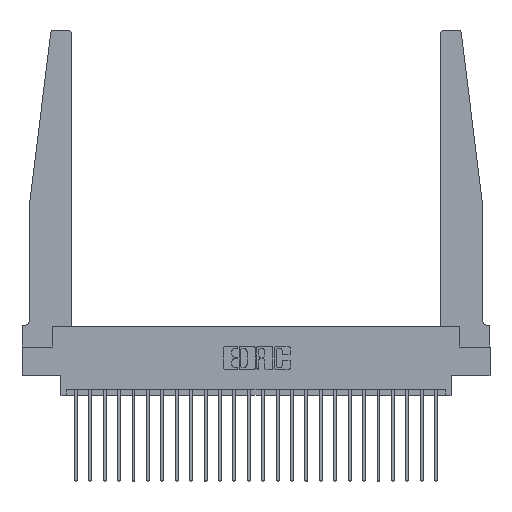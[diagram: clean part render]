
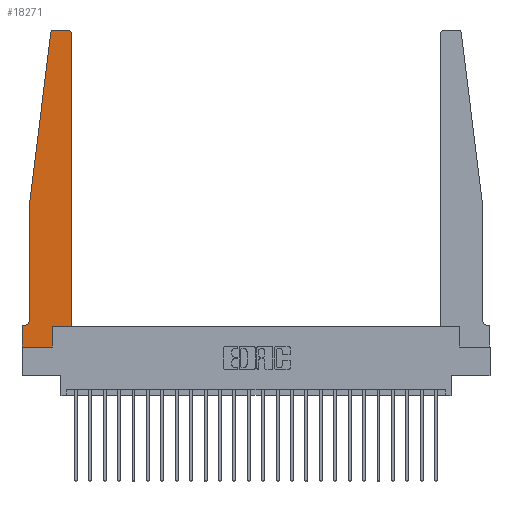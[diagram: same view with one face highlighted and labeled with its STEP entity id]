
A CAD part, top view. The second image highlights one B-rep face of the part: STEP entity #18271.
In plain terms, the highlighted planar face has unit normal (0, 0, 1).
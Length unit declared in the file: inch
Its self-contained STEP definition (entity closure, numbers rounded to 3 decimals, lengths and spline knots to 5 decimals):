
#28 = VECTOR ( 'NONE', #13518, 39.37008 ) ;
#269 = CARTESIAN_POINT ( 'NONE',  ( 0.24675, 2.72367, 0.37 ) ) ;
#648 = ORIENTED_EDGE ( 'NONE', *, *, #5859, .T. ) ;
#719 = CARTESIAN_POINT ( 'NONE',  ( 0., 0., 0.37 ) ) ;
#988 = DIRECTION ( 'NONE',  ( -1., 0., 0. ) ) ;
#1065 = EDGE_CURVE ( 'NONE', #1542, #18862, #12877, .T. ) ;
#1281 = CARTESIAN_POINT ( 'NONE',  ( 0.065, 1.25, 0.37 ) ) ;
#1542 = VERTEX_POINT ( 'NONE', #18149 ) ;
#1634 = CARTESIAN_POINT ( 'NONE',  ( 0.065, 0.1875, 0.37 ) ) ;
#1812 = ORIENTED_EDGE ( 'NONE', *, *, #22918, .T. ) ;
#2038 = EDGE_CURVE ( 'NONE', #8043, #19866, #11413, .T. ) ;
#2056 = EDGE_CURVE ( 'NONE', #17575, #8043, #7572, .T. ) ;
#2084 = ORIENTED_EDGE ( 'NONE', *, *, #17867, .T. ) ;
#2515 = DIRECTION ( 'NONE',  ( 0., 0., 1. ) ) ;
#3106 = VERTEX_POINT ( 'NONE', #269 ) ;
#3423 = DIRECTION ( 'NONE',  ( 0., -1., 0. ) ) ;
#3933 = CARTESIAN_POINT ( 'NONE',  ( 0., 0., 0.37 ) ) ;
#4007 = VECTOR ( 'NONE', #5927, 39.37008 ) ;
#4146 = VECTOR ( 'NONE', #988, 39.37008 ) ;
#4293 = CARTESIAN_POINT ( 'NONE',  ( 0.015, 0.2375, 0.37 ) ) ;
#4571 = ORIENTED_EDGE ( 'NONE', *, *, #20553, .T. ) ;
#5697 = FACE_OUTER_BOUND ( 'NONE', #13056, .T. ) ;
#5859 = EDGE_CURVE ( 'NONE', #18862, #10636, #10485, .T. ) ;
#5927 = DIRECTION ( 'NONE',  ( 1., 0., 0. ) ) ;
#6132 = ORIENTED_EDGE ( 'NONE', *, *, #16201, .T. ) ;
#6278 = DIRECTION ( 'NONE',  ( 1., 0., 0. ) ) ;
#6627 = DIRECTION ( 'NONE',  ( 0., 1., 0. ) ) ;
#6885 = CARTESIAN_POINT ( 'NONE',  ( 0.27653, 2.75, 0.37 ) ) ;
#7199 = ORIENTED_EDGE ( 'NONE', *, *, #8914, .T. ) ;
#7244 = ORIENTED_EDGE ( 'NONE', *, *, #2038, .T. ) ;
#7515 = LINE ( 'NONE', #18513, #19629 ) ;
#7572 = LINE ( 'NONE', #3933, #28 ) ;
#7849 = ORIENTED_EDGE ( 'NONE', *, *, #2056, .T. ) ;
#8014 = CARTESIAN_POINT ( 'NONE',  ( 0.425, 2.72, 0.37 ) ) ;
#8043 = VERTEX_POINT ( 'NONE', #719 ) ;
#8111 = AXIS2_PLACEMENT_3D ( 'NONE', #4293, #11889, #19625 ) ;
#8157 = CARTESIAN_POINT ( 'NONE',  ( 0.395, 2.72, 0.37 ) ) ;
#8914 = EDGE_CURVE ( 'NONE', #11824, #17312, #10185, .T. ) ;
#10185 = CIRCLE ( 'NONE', #19604, 0.03 ) ;
#10283 = VECTOR ( 'NONE', #17275, 39.37008 ) ;
#10485 = CIRCLE ( 'NONE', #8111, 0.05 ) ;
#10636 = VERTEX_POINT ( 'NONE', #20824 ) ;
#11190 = DIRECTION ( 'NONE',  ( 0., 0., 1. ) ) ;
#11413 = LINE ( 'NONE', #20982, #4007 ) ;
#11824 = VERTEX_POINT ( 'NONE', #8014 ) ;
#11889 = DIRECTION ( 'NONE',  ( 0., 0., -1. ) ) ;
#11905 = AXIS2_PLACEMENT_3D ( 'NONE', #17106, #11190, #18698 ) ;
#12877 = LINE ( 'NONE', #1281, #14696 ) ;
#12931 = VECTOR ( 'NONE', #15034, 39.37008 ) ;
#12952 = CARTESIAN_POINT ( 'NONE',  ( 0.425, 0.18, 0.37 ) ) ;
#13056 = EDGE_LOOP ( 'NONE', ( #13083, #1812, #18949, #24376, #648, #6132, #7849, #7244, #15143, #4571, #2084, #7199 ) ) ;
#13083 = ORIENTED_EDGE ( 'NONE', *, *, #21608, .T. ) ;
#13289 = PLANE ( 'NONE',  #11905 ) ;
#13518 = DIRECTION ( 'NONE',  ( 0., -1., 0. ) ) ;
#13530 = EDGE_CURVE ( 'NONE', #3106, #1542, #7515, .T. ) ;
#13970 = CARTESIAN_POINT ( 'NONE',  ( 0.2605, 0., 0.37 ) ) ;
#14323 = CARTESIAN_POINT ( 'NONE',  ( 0.2605, 0.18, 0.37 ) ) ;
#14415 = VECTOR ( 'NONE', #6627, 39.37008 ) ;
#14696 = VECTOR ( 'NONE', #3423, 39.37008 ) ;
#15034 = DIRECTION ( 'NONE',  ( 1., 0., 0. ) ) ;
#15064 = LINE ( 'NONE', #1634, #10283 ) ;
#15143 = ORIENTED_EDGE ( 'NONE', *, *, #22776, .T. ) ;
#15274 = CARTESIAN_POINT ( 'NONE',  ( 0.425, 0.18, 0.37 ) ) ;
#15572 = AXIS2_PLACEMENT_3D ( 'NONE', #16524, #24158, #18601 ) ;
#16201 = EDGE_CURVE ( 'NONE', #10636, #17575, #15064, .T. ) ;
#16524 = CARTESIAN_POINT ( 'NONE',  ( 0.27653, 2.72, 0.37 ) ) ;
#17106 = CARTESIAN_POINT ( 'NONE',  ( 0., 0.1875, 0.37 ) ) ;
#17248 = LINE ( 'NONE', #15274, #21701 ) ;
#17275 = DIRECTION ( 'NONE',  ( -1., 0., 0. ) ) ;
#17312 = VERTEX_POINT ( 'NONE', #24325 ) ;
#17575 = VERTEX_POINT ( 'NONE', #17650 ) ;
#17650 = CARTESIAN_POINT ( 'NONE',  ( 0., 0.1875, 0.37 ) ) ;
#17867 = EDGE_CURVE ( 'NONE', #20613, #11824, #17248, .T. ) ;
#18005 = LINE ( 'NONE', #14323, #14415 ) ;
#18149 = CARTESIAN_POINT ( 'NONE',  ( 0.065, 1.25, 0.37 ) ) ;
#18271 = ADVANCED_FACE ( 'NONE', ( #5697 ), #13289, .T. ) ;
#18513 = CARTESIAN_POINT ( 'NONE',  ( 0.065, 1.25, 0.37 ) ) ;
#18601 = DIRECTION ( 'NONE',  ( 1., 0., 0. ) ) ;
#18698 = DIRECTION ( 'NONE',  ( 1., 0., 0. ) ) ;
#18714 = CARTESIAN_POINT ( 'NONE',  ( 0.425, 0.18, 0.37 ) ) ;
#18739 = VERTEX_POINT ( 'NONE', #22701 ) ;
#18862 = VERTEX_POINT ( 'NONE', #23137 ) ;
#18949 = ORIENTED_EDGE ( 'NONE', *, *, #13530, .T. ) ;
#19604 = AXIS2_PLACEMENT_3D ( 'NONE', #8157, #2515, #6278 ) ;
#19625 = DIRECTION ( 'NONE',  ( -1., 0., 0. ) ) ;
#19629 = VECTOR ( 'NONE', #20567, 39.37008 ) ;
#19866 = VERTEX_POINT ( 'NONE', #13970 ) ;
#20553 = EDGE_CURVE ( 'NONE', #18739, #20613, #24042, .T. ) ;
#20567 = DIRECTION ( 'NONE',  ( -0.122, -0.992, 0. ) ) ;
#20613 = VERTEX_POINT ( 'NONE', #12952 ) ;
#20643 = CIRCLE ( 'NONE', #15572, 0.03 ) ;
#20824 = CARTESIAN_POINT ( 'NONE',  ( 0.015, 0.1875, 0.37 ) ) ;
#20909 = DIRECTION ( 'NONE',  ( 0., 1., 0. ) ) ;
#20982 = CARTESIAN_POINT ( 'NONE',  ( 0., 0., 0.37 ) ) ;
#21100 = VERTEX_POINT ( 'NONE', #6885 ) ;
#21608 = EDGE_CURVE ( 'NONE', #17312, #21100, #23786, .T. ) ;
#21671 = CARTESIAN_POINT ( 'NONE',  ( 0.25, 2.75, 0.37 ) ) ;
#21701 = VECTOR ( 'NONE', #20909, 39.37008 ) ;
#22701 = CARTESIAN_POINT ( 'NONE',  ( 0.2605, 0.18, 0.37 ) ) ;
#22776 = EDGE_CURVE ( 'NONE', #19866, #18739, #18005, .T. ) ;
#22918 = EDGE_CURVE ( 'NONE', #21100, #3106, #20643, .T. ) ;
#23137 = CARTESIAN_POINT ( 'NONE',  ( 0.065, 0.2375, 0.37 ) ) ;
#23786 = LINE ( 'NONE', #21671, #4146 ) ;
#24042 = LINE ( 'NONE', #18714, #12931 ) ;
#24158 = DIRECTION ( 'NONE',  ( 0., 0., 1. ) ) ;
#24325 = CARTESIAN_POINT ( 'NONE',  ( 0.395, 2.75, 0.37 ) ) ;
#24376 = ORIENTED_EDGE ( 'NONE', *, *, #1065, .T. ) ;
